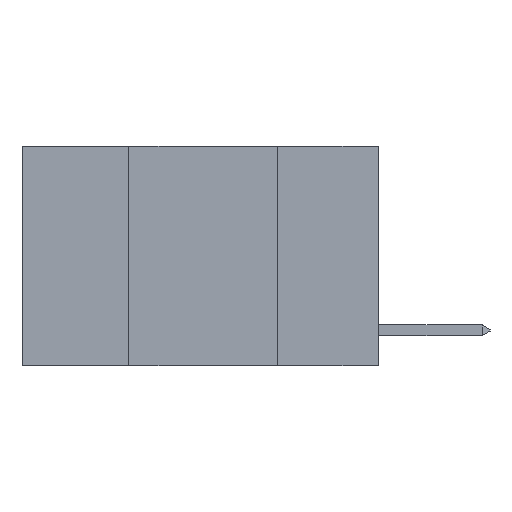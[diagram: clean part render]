
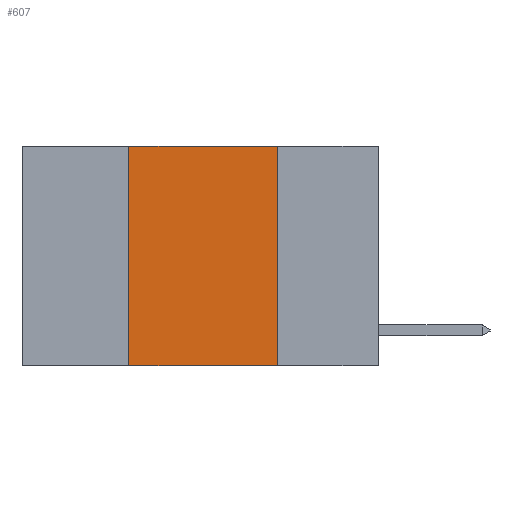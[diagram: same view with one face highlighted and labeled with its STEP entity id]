
A CAD part, left-side view. The second image highlights one B-rep face of the part: STEP entity #607.
In plain terms, the highlighted planar face has unit normal (-1, 0, 0).
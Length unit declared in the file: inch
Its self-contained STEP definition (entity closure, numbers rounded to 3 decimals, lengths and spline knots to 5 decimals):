
#180 = DIRECTION ( 'NONE',  ( 0., 0., -1. ) ) ;
#228 = DIRECTION ( 'NONE',  ( 1., 0., 0. ) ) ;
#296 = PLANE ( 'NONE',  #1911 ) ;
#451 = LINE ( 'NONE', #1674, #8226 ) ;
#550 = CARTESIAN_POINT ( 'NONE',  ( 0., 0.6, 0. ) ) ;
#607 = ADVANCED_FACE ( 'NONE', ( #4479 ), #296, .F. ) ;
#843 = DIRECTION ( 'NONE',  ( 0., 0., 1. ) ) ;
#1674 = CARTESIAN_POINT ( 'NONE',  ( 0., 0.6, 0. ) ) ;
#1911 = AXIS2_PLACEMENT_3D ( 'NONE', #550, #228, #180 ) ;
#2101 = DIRECTION ( 'NONE',  ( 0., -1., 0. ) ) ;
#2681 = DIRECTION ( 'NONE',  ( 0., -1., 0. ) ) ;
#2767 = CARTESIAN_POINT ( 'NONE',  ( 0., 0.17, 0. ) ) ;
#3331 = CARTESIAN_POINT ( 'NONE',  ( 0., 0.42, 0. ) ) ;
#3633 = VERTEX_POINT ( 'NONE', #9214 ) ;
#3809 = EDGE_CURVE ( 'NONE', #12285, #3633, #4566, .T. ) ;
#3923 = CARTESIAN_POINT ( 'NONE',  ( 0., 0.42, -0.37 ) ) ;
#3967 = VERTEX_POINT ( 'NONE', #3923 ) ;
#4220 = ORIENTED_EDGE ( 'NONE', *, *, #3809, .F. ) ;
#4244 = ORIENTED_EDGE ( 'NONE', *, *, #11412, .F. ) ;
#4479 = FACE_OUTER_BOUND ( 'NONE', #9991, .T. ) ;
#4566 = LINE ( 'NONE', #2767, #7439 ) ;
#5067 = VECTOR ( 'NONE', #843, 39.37008 ) ;
#5068 = ORIENTED_EDGE ( 'NONE', *, *, #6756, .F. ) ;
#5097 = ORIENTED_EDGE ( 'NONE', *, *, #12171, .T. ) ;
#5685 = LINE ( 'NONE', #5792, #5067 ) ;
#5792 = CARTESIAN_POINT ( 'NONE',  ( 0., 0.42, 0. ) ) ;
#6756 = EDGE_CURVE ( 'NONE', #3967, #9387, #5685, .T. ) ;
#6807 = VECTOR ( 'NONE', #2101, 39.37008 ) ;
#7439 = VECTOR ( 'NONE', #9467, 39.37008 ) ;
#8226 = VECTOR ( 'NONE', #2681, 39.37008 ) ;
#9214 = CARTESIAN_POINT ( 'NONE',  ( 0., 0.17, -0.37 ) ) ;
#9387 = VERTEX_POINT ( 'NONE', #3331 ) ;
#9467 = DIRECTION ( 'NONE',  ( 0., 0., -1. ) ) ;
#9548 = LINE ( 'NONE', #10665, #6807 ) ;
#9991 = EDGE_LOOP ( 'NONE', ( #4220, #4244, #5068, #5097 ) ) ;
#10665 = CARTESIAN_POINT ( 'NONE',  ( 0., 0.6, -0.37 ) ) ;
#10828 = CARTESIAN_POINT ( 'NONE',  ( 0., 0.17, 0. ) ) ;
#11412 = EDGE_CURVE ( 'NONE', #9387, #12285, #451, .T. ) ;
#12171 = EDGE_CURVE ( 'NONE', #3967, #3633, #9548, .T. ) ;
#12285 = VERTEX_POINT ( 'NONE', #10828 ) ;
